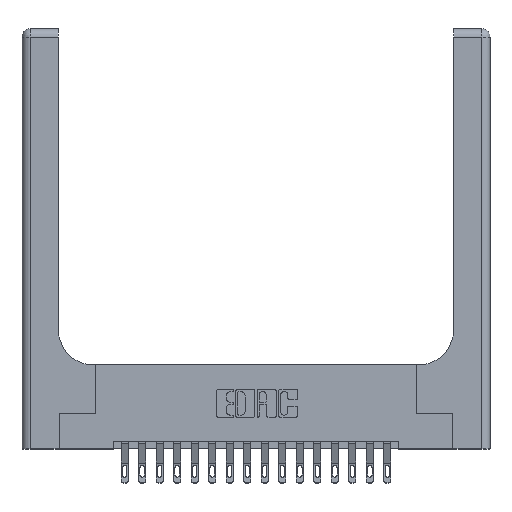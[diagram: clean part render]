
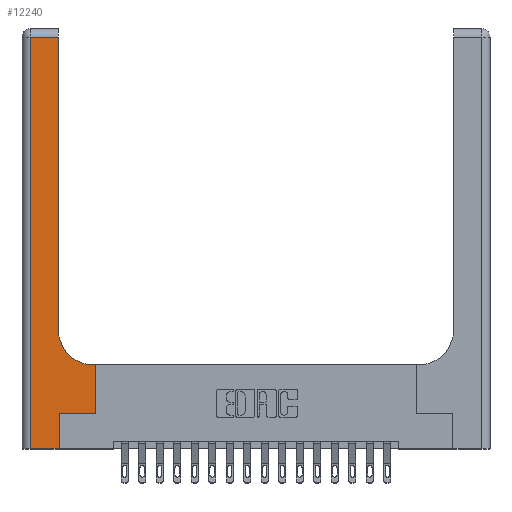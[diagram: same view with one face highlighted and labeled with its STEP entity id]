
A CAD part, top view. The second image highlights one B-rep face of the part: STEP entity #12240.
In plain terms, the highlighted planar face has unit normal (0, 0, 1).
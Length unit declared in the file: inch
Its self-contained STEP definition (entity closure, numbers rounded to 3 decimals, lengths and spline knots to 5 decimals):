
#102 = CARTESIAN_POINT ( 'NONE',  ( 0.265, 0., 0.37 ) ) ;
#299 = CARTESIAN_POINT ( 'NONE',  ( 0.06, 2.94, 0.37 ) ) ;
#493 = ORIENTED_EDGE ( 'NONE', *, *, #1856, .T. ) ;
#808 = AXIS2_PLACEMENT_3D ( 'NONE', #14469, #15854, #11358 ) ;
#1055 = LINE ( 'NONE', #7218, #3496 ) ;
#1162 = VERTEX_POINT ( 'NONE', #19850 ) ;
#1165 = VERTEX_POINT ( 'NONE', #18441 ) ;
#1194 = EDGE_CURVE ( 'NONE', #19583, #15084, #10697, .T. ) ;
#1266 = VERTEX_POINT ( 'NONE', #6572 ) ;
#1435 = CIRCLE ( 'NONE', #808, 0.25 ) ;
#1559 = ORIENTED_EDGE ( 'NONE', *, *, #12426, .T. ) ;
#1564 = EDGE_CURVE ( 'NONE', #15084, #5491, #1435, .T. ) ;
#1856 = EDGE_CURVE ( 'NONE', #10450, #6704, #6296, .T. ) ;
#1915 = AXIS2_PLACEMENT_3D ( 'NONE', #10830, #8022, #9228 ) ;
#1955 = CARTESIAN_POINT ( 'NONE',  ( 0.528, 0.25, 0.37 ) ) ;
#2675 = ORIENTED_EDGE ( 'NONE', *, *, #1194, .T. ) ;
#2697 = VECTOR ( 'NONE', #10624, 39.37008 ) ;
#3120 = DIRECTION ( 'NONE',  ( 0., 1., 0. ) ) ;
#3496 = VECTOR ( 'NONE', #13173, 39.37008 ) ;
#4332 = ORIENTED_EDGE ( 'NONE', *, *, #11008, .T. ) ;
#4427 = ORIENTED_EDGE ( 'NONE', *, *, #13946, .T. ) ;
#4984 = ORIENTED_EDGE ( 'NONE', *, *, #15447, .T. ) ;
#5090 = EDGE_CURVE ( 'NONE', #1165, #1266, #10783, .T. ) ;
#5491 = VERTEX_POINT ( 'NONE', #10763 ) ;
#5805 = CARTESIAN_POINT ( 'NONE',  ( 0.528, 0.6, 0.37 ) ) ;
#5886 = VECTOR ( 'NONE', #12323, 39.37008 ) ;
#6194 = CARTESIAN_POINT ( 'NONE',  ( 0.06, 3., 0.37 ) ) ;
#6296 = LINE ( 'NONE', #6194, #2697 ) ;
#6304 = FACE_OUTER_BOUND ( 'NONE', #11669, .T. ) ;
#6572 = CARTESIAN_POINT ( 'NONE',  ( 0.265, 0.25, 0.37 ) ) ;
#6600 = CARTESIAN_POINT ( 'NONE',  ( 0., 0., 0.37 ) ) ;
#6704 = VERTEX_POINT ( 'NONE', #17165 ) ;
#6794 = VECTOR ( 'NONE', #17922, 39.37008 ) ;
#6842 = VECTOR ( 'NONE', #3120, 39.37008 ) ;
#7218 = CARTESIAN_POINT ( 'NONE',  ( 0., 2.94, 0.37 ) ) ;
#7481 = CARTESIAN_POINT ( 'NONE',  ( 0.51, 0.6, 0.37 ) ) ;
#7692 = CARTESIAN_POINT ( 'NONE',  ( 0.26, 0.6, 0.37 ) ) ;
#8022 = DIRECTION ( 'NONE',  ( 0., 0., -1. ) ) ;
#8116 = LINE ( 'NONE', #6600, #11764 ) ;
#8221 = LINE ( 'NONE', #1955, #16691 ) ;
#8354 = EDGE_CURVE ( 'NONE', #6704, #1165, #8116, .T. ) ;
#8685 = CARTESIAN_POINT ( 'NONE',  ( 0.26, 3., 0.37 ) ) ;
#9228 = DIRECTION ( 'NONE',  ( -1., 0., 0. ) ) ;
#10177 = LINE ( 'NONE', #18005, #11348 ) ;
#10450 = VERTEX_POINT ( 'NONE', #299 ) ;
#10624 = DIRECTION ( 'NONE',  ( 0., -1., 0. ) ) ;
#10697 = LINE ( 'NONE', #7692, #5886 ) ;
#10763 = CARTESIAN_POINT ( 'NONE',  ( 0.26, 0.85, 0.37 ) ) ;
#10783 = LINE ( 'NONE', #102, #6842 ) ;
#10830 = CARTESIAN_POINT ( 'NONE',  ( 0., 3., 0.37 ) ) ;
#11008 = EDGE_CURVE ( 'NONE', #1162, #10450, #1055, .T. ) ;
#11348 = VECTOR ( 'NONE', #16376, 39.37008 ) ;
#11358 = DIRECTION ( 'NONE',  ( 1., 0., 0. ) ) ;
#11669 = EDGE_LOOP ( 'NONE', ( #4427, #4332, #493, #11862, #16424, #4984, #1559, #2675, #14017 ) ) ;
#11764 = VECTOR ( 'NONE', #18868, 39.37008 ) ;
#11862 = ORIENTED_EDGE ( 'NONE', *, *, #8354, .T. ) ;
#12205 = CARTESIAN_POINT ( 'NONE',  ( 0.528, 0.25, 0.37 ) ) ;
#12240 = ADVANCED_FACE ( 'NONE', ( #6304 ), #15257, .F. ) ;
#12323 = DIRECTION ( 'NONE',  ( -1., 0., 0. ) ) ;
#12426 = EDGE_CURVE ( 'NONE', #13104, #19583, #8221, .T. ) ;
#13104 = VERTEX_POINT ( 'NONE', #12205 ) ;
#13173 = DIRECTION ( 'NONE',  ( -1., 0., 0. ) ) ;
#13946 = EDGE_CURVE ( 'NONE', #5491, #1162, #19639, .T. ) ;
#14017 = ORIENTED_EDGE ( 'NONE', *, *, #1564, .T. ) ;
#14469 = CARTESIAN_POINT ( 'NONE',  ( 0.51, 0.85, 0.37 ) ) ;
#15084 = VERTEX_POINT ( 'NONE', #7481 ) ;
#15257 = PLANE ( 'NONE',  #1915 ) ;
#15447 = EDGE_CURVE ( 'NONE', #1266, #13104, #10177, .T. ) ;
#15854 = DIRECTION ( 'NONE',  ( 0., 0., -1. ) ) ;
#16376 = DIRECTION ( 'NONE',  ( 1., 0., 0. ) ) ;
#16424 = ORIENTED_EDGE ( 'NONE', *, *, #5090, .T. ) ;
#16691 = VECTOR ( 'NONE', #18874, 39.37008 ) ;
#17165 = CARTESIAN_POINT ( 'NONE',  ( 0.06, 0., 0.37 ) ) ;
#17922 = DIRECTION ( 'NONE',  ( 0., 1., 0. ) ) ;
#18005 = CARTESIAN_POINT ( 'NONE',  ( 0.265, 0.25, 0.37 ) ) ;
#18441 = CARTESIAN_POINT ( 'NONE',  ( 0.265, 0., 0.37 ) ) ;
#18868 = DIRECTION ( 'NONE',  ( 1., 0., 0. ) ) ;
#18874 = DIRECTION ( 'NONE',  ( 0., 1., 0. ) ) ;
#19583 = VERTEX_POINT ( 'NONE', #5805 ) ;
#19639 = LINE ( 'NONE', #8685, #6794 ) ;
#19850 = CARTESIAN_POINT ( 'NONE',  ( 0.26, 2.94, 0.37 ) ) ;
